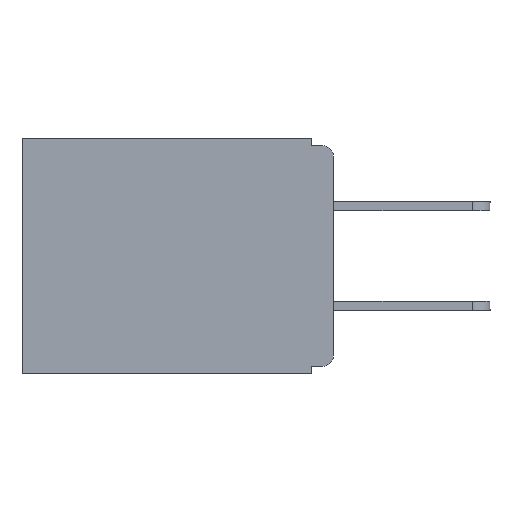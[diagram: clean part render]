
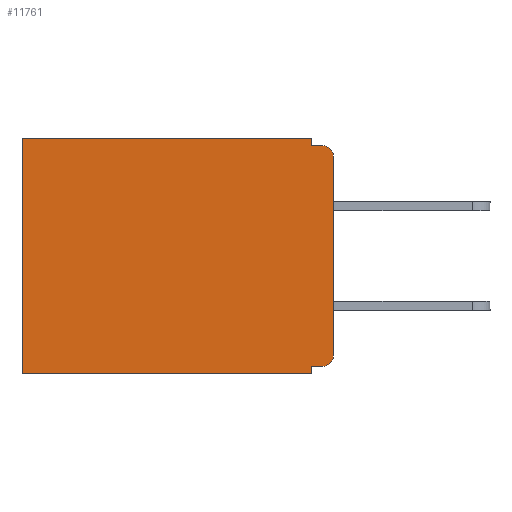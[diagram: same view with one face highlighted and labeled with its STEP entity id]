
A CAD part, left-side view. The second image highlights one B-rep face of the part: STEP entity #11761.
In plain terms, the highlighted planar face has unit normal (-1, 0, 0).
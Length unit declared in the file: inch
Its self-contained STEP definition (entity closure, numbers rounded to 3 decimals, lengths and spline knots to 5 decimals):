
#479 = CARTESIAN_POINT ( 'NONE',  ( 0.3, 0.437, -0.33 ) ) ;
#563 = CARTESIAN_POINT ( 'NONE',  ( 0.3, 0.015, -0.01 ) ) ;
#786 = CARTESIAN_POINT ( 'NONE',  ( 0.3, 0.031, -0.33 ) ) ;
#848 = CARTESIAN_POINT ( 'NONE',  ( 0.3, 0.031, 0. ) ) ;
#929 = EDGE_CURVE ( 'NONE', #4433, #4142, #8367, .T. ) ;
#1148 = VERTEX_POINT ( 'NONE', #479 ) ;
#1218 = EDGE_CURVE ( 'NONE', #11671, #6593, #6511, .T. ) ;
#1223 = DIRECTION ( 'NONE',  ( -1., 0., 0. ) ) ;
#1251 = EDGE_CURVE ( 'NONE', #2166, #4142, #6311, .T. ) ;
#1385 = EDGE_CURVE ( 'NONE', #11671, #6457, #6030, .T. ) ;
#1515 = LINE ( 'NONE', #2636, #1543 ) ;
#1543 = VECTOR ( 'NONE', #10200, 39.37008 ) ;
#1992 = EDGE_CURVE ( 'NONE', #3038, #4785, #5339, .T. ) ;
#2112 = DIRECTION ( 'NONE',  ( 0., 0., -1. ) ) ;
#2163 = EDGE_LOOP ( 'NONE', ( #9530, #2985, #2976, #9651, #2864, #2809, #9666, #3161, #3139, #9678 ) ) ;
#2166 = VERTEX_POINT ( 'NONE', #10793 ) ;
#2636 = CARTESIAN_POINT ( 'NONE',  ( 0.3, 0., -0.33 ) ) ;
#2809 = ORIENTED_EDGE ( 'NONE', *, *, #2842, .T. ) ;
#2842 = EDGE_CURVE ( 'NONE', #4785, #1148, #6596, .T. ) ;
#2864 = ORIENTED_EDGE ( 'NONE', *, *, #1992, .T. ) ;
#2976 = ORIENTED_EDGE ( 'NONE', *, *, #929, .F. ) ;
#2985 = ORIENTED_EDGE ( 'NONE', *, *, #1251, .T. ) ;
#3038 = VERTEX_POINT ( 'NONE', #4903 ) ;
#3139 = ORIENTED_EDGE ( 'NONE', *, *, #1218, .F. ) ;
#3161 = ORIENTED_EDGE ( 'NONE', *, *, #4199, .F. ) ;
#3523 = DIRECTION ( 'NONE',  ( -1., 0., 0. ) ) ;
#3616 = EDGE_CURVE ( 'NONE', #7413, #1148, #1515, .T. ) ;
#3985 = CARTESIAN_POINT ( 'NONE',  ( 0.3, 0.437, -0.33 ) ) ;
#4118 = EDGE_CURVE ( 'NONE', #3038, #4433, #9990, .T. ) ;
#4142 = VERTEX_POINT ( 'NONE', #563 ) ;
#4199 = EDGE_CURVE ( 'NONE', #6593, #7413, #9104, .T. ) ;
#4433 = VERTEX_POINT ( 'NONE', #11577 ) ;
#4785 = VERTEX_POINT ( 'NONE', #10644 ) ;
#4903 = CARTESIAN_POINT ( 'NONE',  ( 0.3, 0.031, 0. ) ) ;
#5220 = CARTESIAN_POINT ( 'NONE',  ( 0.3, 0., -0.33 ) ) ;
#5236 = DIRECTION ( 'NONE',  ( 0., 0., -1. ) ) ;
#5270 = VECTOR ( 'NONE', #8775, 39.37008 ) ;
#5339 = LINE ( 'NONE', #8233, #5270 ) ;
#5904 = CARTESIAN_POINT ( 'NONE',  ( 0.3, 0.031, -0.33 ) ) ;
#6030 = CIRCLE ( 'NONE', #11221, 0.015 ) ;
#6311 = CIRCLE ( 'NONE', #7560, 0.015 ) ;
#6442 = VECTOR ( 'NONE', #9170, 39.37008 ) ;
#6457 = VERTEX_POINT ( 'NONE', #9459 ) ;
#6511 = LINE ( 'NONE', #10203, #6442 ) ;
#6593 = VERTEX_POINT ( 'NONE', #8399 ) ;
#6596 = LINE ( 'NONE', #3985, #6745 ) ;
#6745 = VECTOR ( 'NONE', #8474, 39.37008 ) ;
#7413 = VERTEX_POINT ( 'NONE', #5904 ) ;
#7560 = AXIS2_PLACEMENT_3D ( 'NONE', #8604, #3523, #2112 ) ;
#7776 = VECTOR ( 'NONE', #8796, 39.37008 ) ;
#8054 = VECTOR ( 'NONE', #5236, 39.37008 ) ;
#8198 = LINE ( 'NONE', #5220, #8054 ) ;
#8233 = CARTESIAN_POINT ( 'NONE',  ( 0.3, 0., 0. ) ) ;
#8320 = DIRECTION ( 'NONE',  ( 0., 0., -1. ) ) ;
#8367 = LINE ( 'NONE', #11632, #7776 ) ;
#8399 = CARTESIAN_POINT ( 'NONE',  ( 0.3, 0.031, -0.32 ) ) ;
#8474 = DIRECTION ( 'NONE',  ( 0., 0., -1. ) ) ;
#8604 = CARTESIAN_POINT ( 'NONE',  ( 0.3, 0.015, -0.025 ) ) ;
#8734 = VECTOR ( 'NONE', #8762, 39.37008 ) ;
#8762 = DIRECTION ( 'NONE',  ( 0., 0., -1. ) ) ;
#8775 = DIRECTION ( 'NONE',  ( 0., 1., 0. ) ) ;
#8796 = DIRECTION ( 'NONE',  ( 0., -1., 0. ) ) ;
#8862 = AXIS2_PLACEMENT_3D ( 'NONE', #10486, #10347, #10310 ) ;
#8880 = FACE_OUTER_BOUND ( 'NONE', #2163, .T. ) ;
#9104 = LINE ( 'NONE', #786, #8734 ) ;
#9170 = DIRECTION ( 'NONE',  ( 0., 1., 0. ) ) ;
#9459 = CARTESIAN_POINT ( 'NONE',  ( 0.3, 0., -0.305 ) ) ;
#9467 = EDGE_CURVE ( 'NONE', #2166, #6457, #8198, .T. ) ;
#9530 = ORIENTED_EDGE ( 'NONE', *, *, #9467, .F. ) ;
#9651 = ORIENTED_EDGE ( 'NONE', *, *, #4118, .F. ) ;
#9666 = ORIENTED_EDGE ( 'NONE', *, *, #3616, .F. ) ;
#9678 = ORIENTED_EDGE ( 'NONE', *, *, #1385, .T. ) ;
#9990 = LINE ( 'NONE', #848, #10210 ) ;
#10200 = DIRECTION ( 'NONE',  ( 0., 1., 0. ) ) ;
#10203 = CARTESIAN_POINT ( 'NONE',  ( 0.3, 0., -0.32 ) ) ;
#10210 = VECTOR ( 'NONE', #8320, 39.37008 ) ;
#10310 = DIRECTION ( 'NONE',  ( 0., 0., -1. ) ) ;
#10347 = DIRECTION ( 'NONE',  ( 1., 0., 0. ) ) ;
#10486 = CARTESIAN_POINT ( 'NONE',  ( 0.3, 0., -0.33 ) ) ;
#10568 = PLANE ( 'NONE',  #8862 ) ;
#10644 = CARTESIAN_POINT ( 'NONE',  ( 0.3, 0.437, 0. ) ) ;
#10793 = CARTESIAN_POINT ( 'NONE',  ( 0.3, 0., -0.025 ) ) ;
#11148 = CARTESIAN_POINT ( 'NONE',  ( 0.3, 0.015, -0.32 ) ) ;
#11221 = AXIS2_PLACEMENT_3D ( 'NONE', #11704, #1223, #11615 ) ;
#11577 = CARTESIAN_POINT ( 'NONE',  ( 0.3, 0.031, -0.01 ) ) ;
#11615 = DIRECTION ( 'NONE',  ( 0., 0., -1. ) ) ;
#11632 = CARTESIAN_POINT ( 'NONE',  ( 0.3, 0., -0.01 ) ) ;
#11671 = VERTEX_POINT ( 'NONE', #11148 ) ;
#11704 = CARTESIAN_POINT ( 'NONE',  ( 0.3, 0.015, -0.305 ) ) ;
#11761 = ADVANCED_FACE ( 'NONE', ( #8880 ), #10568, .F. ) ;
